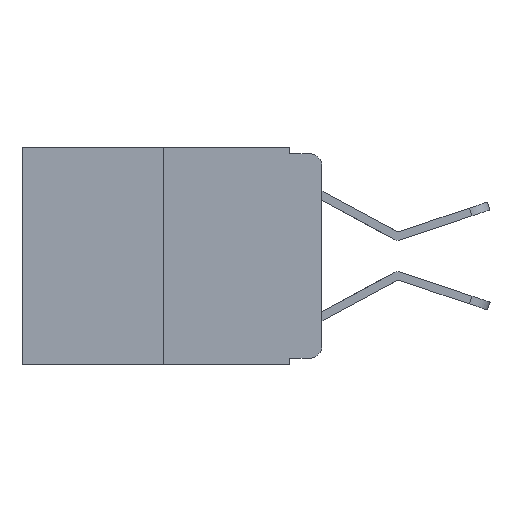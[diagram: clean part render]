
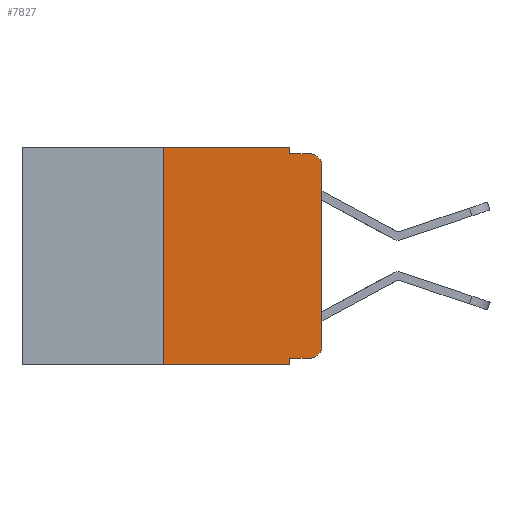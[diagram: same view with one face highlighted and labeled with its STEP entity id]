
A CAD part, left-side view. The second image highlights one B-rep face of the part: STEP entity #7827.
In plain terms, the highlighted planar face has unit normal (-1, 0, 0).
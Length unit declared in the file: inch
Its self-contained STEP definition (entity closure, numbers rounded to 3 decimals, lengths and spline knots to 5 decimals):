
#40 = ORIENTED_EDGE ( 'NONE', *, *, #6646, .F. ) ;
#112 = CARTESIAN_POINT ( 'NONE',  ( 0., 0.051, 0. ) ) ;
#167 = CARTESIAN_POINT ( 'NONE',  ( 0., 0.051, -0.01 ) ) ;
#437 = CIRCLE ( 'NONE', #8826, 0.02 ) ;
#723 = FACE_OUTER_BOUND ( 'NONE', #4966, .T. ) ;
#824 = DIRECTION ( 'NONE',  ( -1., 0., 0. ) ) ;
#918 = VECTOR ( 'NONE', #6044, 39.37008 ) ;
#944 = CARTESIAN_POINT ( 'NONE',  ( 0., 0.02, -0.01 ) ) ;
#1312 = EDGE_CURVE ( 'NONE', #7661, #6395, #2126, .T. ) ;
#1592 = ORIENTED_EDGE ( 'NONE', *, *, #10351, .F. ) ;
#1597 = VECTOR ( 'NONE', #8330, 39.37008 ) ;
#1620 = VECTOR ( 'NONE', #2659, 39.37008 ) ;
#1896 = LINE ( 'NONE', #4567, #6609 ) ;
#2082 = EDGE_CURVE ( 'NONE', #5813, #6395, #437, .T. ) ;
#2126 = LINE ( 'NONE', #10202, #2555 ) ;
#2179 = DIRECTION ( 'NONE',  ( 0., 0., -1. ) ) ;
#2227 = EDGE_CURVE ( 'NONE', #5006, #5813, #6166, .T. ) ;
#2341 = ORIENTED_EDGE ( 'NONE', *, *, #3551, .T. ) ;
#2454 = CARTESIAN_POINT ( 'NONE',  ( 0., 0.25, 0. ) ) ;
#2528 = CARTESIAN_POINT ( 'NONE',  ( 0., 0.02, -0.333 ) ) ;
#2536 = VERTEX_POINT ( 'NONE', #3387 ) ;
#2555 = VECTOR ( 'NONE', #3324, 39.37008 ) ;
#2566 = DIRECTION ( 'NONE',  ( 1., 0., 0. ) ) ;
#2575 = EDGE_CURVE ( 'NONE', #6196, #2536, #3357, .T. ) ;
#2593 = CARTESIAN_POINT ( 'NONE',  ( 0., 0.02, -0.03 ) ) ;
#2659 = DIRECTION ( 'NONE',  ( 0., 0., 1. ) ) ;
#3324 = DIRECTION ( 'NONE',  ( 0., -1., 0. ) ) ;
#3357 = LINE ( 'NONE', #4015, #10318 ) ;
#3387 = CARTESIAN_POINT ( 'NONE',  ( 0., 0.051, -0.343 ) ) ;
#3438 = DIRECTION ( 'NONE',  ( 0., 0., -1. ) ) ;
#3446 = VERTEX_POINT ( 'NONE', #9344 ) ;
#3533 = ORIENTED_EDGE ( 'NONE', *, *, #7927, .T. ) ;
#3551 = EDGE_CURVE ( 'NONE', #6568, #4152, #9879, .T. ) ;
#3924 = DIRECTION ( 'NONE',  ( 0., -1., 0. ) ) ;
#4015 = CARTESIAN_POINT ( 'NONE',  ( 0., 0.473, -0.343 ) ) ;
#4152 = VERTEX_POINT ( 'NONE', #2528 ) ;
#4326 = VERTEX_POINT ( 'NONE', #112 ) ;
#4342 = LINE ( 'NONE', #5149, #918 ) ;
#4475 = CARTESIAN_POINT ( 'NONE',  ( 0., 0.02, -0.313 ) ) ;
#4567 = CARTESIAN_POINT ( 'NONE',  ( 0., 0.051, 0. ) ) ;
#4862 = CARTESIAN_POINT ( 'NONE',  ( 0., 0.051, -0.333 ) ) ;
#4944 = ORIENTED_EDGE ( 'NONE', *, *, #2082, .T. ) ;
#4966 = EDGE_LOOP ( 'NONE', ( #8571, #4944, #10211, #7619, #1592, #9790, #7359, #40, #2341, #3533 ) ) ;
#5006 = VERTEX_POINT ( 'NONE', #10800 ) ;
#5149 = CARTESIAN_POINT ( 'NONE',  ( 0., 0.051, 0. ) ) ;
#5513 = CARTESIAN_POINT ( 'NONE',  ( 0., 0.473, 0. ) ) ;
#5564 = DIRECTION ( 'NONE',  ( 0., 0., -1. ) ) ;
#5681 = LINE ( 'NONE', #2454, #8211 ) ;
#5813 = VERTEX_POINT ( 'NONE', #9888 ) ;
#6044 = DIRECTION ( 'NONE',  ( 0., 0., -1. ) ) ;
#6150 = AXIS2_PLACEMENT_3D ( 'NONE', #7739, #2566, #3438 ) ;
#6166 = LINE ( 'NONE', #10320, #1620 ) ;
#6196 = VERTEX_POINT ( 'NONE', #10980 ) ;
#6395 = VERTEX_POINT ( 'NONE', #944 ) ;
#6429 = DIRECTION ( 'NONE',  ( 0., -1., 0. ) ) ;
#6568 = VERTEX_POINT ( 'NONE', #7230 ) ;
#6609 = VECTOR ( 'NONE', #5564, 39.37008 ) ;
#6646 = EDGE_CURVE ( 'NONE', #6568, #2536, #1896, .T. ) ;
#7230 = CARTESIAN_POINT ( 'NONE',  ( 0., 0.051, -0.333 ) ) ;
#7305 = VECTOR ( 'NONE', #3924, 39.37008 ) ;
#7359 = ORIENTED_EDGE ( 'NONE', *, *, #2575, .T. ) ;
#7416 = EDGE_CURVE ( 'NONE', #6196, #3446, #5681, .T. ) ;
#7519 = CIRCLE ( 'NONE', #8662, 0.02 ) ;
#7619 = ORIENTED_EDGE ( 'NONE', *, *, #9986, .F. ) ;
#7661 = VERTEX_POINT ( 'NONE', #167 ) ;
#7704 = PLANE ( 'NONE',  #6150 ) ;
#7739 = CARTESIAN_POINT ( 'NONE',  ( 0., 0.473, 0. ) ) ;
#7827 = ADVANCED_FACE ( 'NONE', ( #723 ), #7704, .F. ) ;
#7927 = EDGE_CURVE ( 'NONE', #4152, #5006, #7519, .T. ) ;
#8211 = VECTOR ( 'NONE', #10021, 39.37008 ) ;
#8330 = DIRECTION ( 'NONE',  ( 0., -1., 0. ) ) ;
#8571 = ORIENTED_EDGE ( 'NONE', *, *, #2227, .T. ) ;
#8662 = AXIS2_PLACEMENT_3D ( 'NONE', #4475, #10461, #2179 ) ;
#8826 = AXIS2_PLACEMENT_3D ( 'NONE', #2593, #824, #10301 ) ;
#9344 = CARTESIAN_POINT ( 'NONE',  ( 0., 0.25, 0. ) ) ;
#9578 = LINE ( 'NONE', #5513, #7305 ) ;
#9790 = ORIENTED_EDGE ( 'NONE', *, *, #7416, .F. ) ;
#9879 = LINE ( 'NONE', #4862, #1597 ) ;
#9888 = CARTESIAN_POINT ( 'NONE',  ( 0., 0., -0.03 ) ) ;
#9986 = EDGE_CURVE ( 'NONE', #4326, #7661, #4342, .T. ) ;
#10021 = DIRECTION ( 'NONE',  ( 0., 0., 1. ) ) ;
#10202 = CARTESIAN_POINT ( 'NONE',  ( 0., 0.051, -0.01 ) ) ;
#10211 = ORIENTED_EDGE ( 'NONE', *, *, #1312, .F. ) ;
#10301 = DIRECTION ( 'NONE',  ( 0., 0., -1. ) ) ;
#10318 = VECTOR ( 'NONE', #6429, 39.37008 ) ;
#10320 = CARTESIAN_POINT ( 'NONE',  ( 0., 0., 0. ) ) ;
#10351 = EDGE_CURVE ( 'NONE', #3446, #4326, #9578, .T. ) ;
#10461 = DIRECTION ( 'NONE',  ( -1., 0., 0. ) ) ;
#10800 = CARTESIAN_POINT ( 'NONE',  ( 0., 0., -0.313 ) ) ;
#10980 = CARTESIAN_POINT ( 'NONE',  ( 0., 0.25, -0.343 ) ) ;
